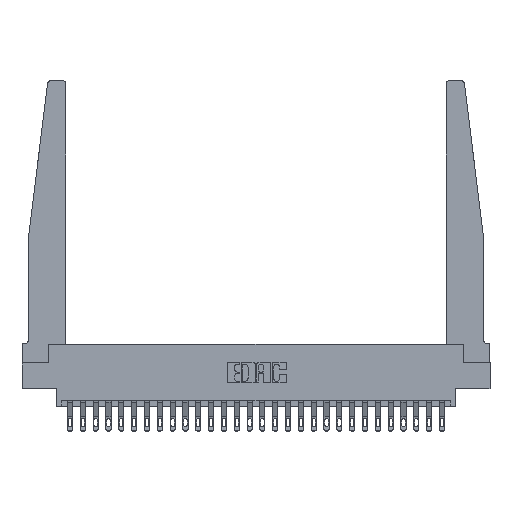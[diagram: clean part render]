
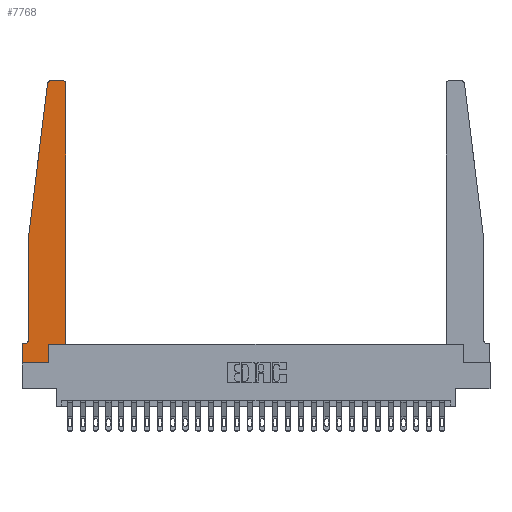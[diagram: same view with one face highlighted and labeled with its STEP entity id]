
A CAD part, top view. The second image highlights one B-rep face of the part: STEP entity #7768.
In plain terms, the highlighted planar face has unit normal (0, 0, 1).
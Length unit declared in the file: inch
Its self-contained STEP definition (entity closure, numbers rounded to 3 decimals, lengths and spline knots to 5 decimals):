
#263 = LINE ( 'NONE', #19004, #9302 ) ;
#421 = LINE ( 'NONE', #19478, #10753 ) ;
#685 = ORIENTED_EDGE ( 'NONE', *, *, #16748, .T. ) ;
#1182 = CARTESIAN_POINT ( 'NONE',  ( 0., 0., 0.37 ) ) ;
#1419 = EDGE_CURVE ( 'NONE', #20278, #16395, #15448, .T. ) ;
#1498 = ORIENTED_EDGE ( 'NONE', *, *, #15042, .T. ) ;
#1793 = EDGE_CURVE ( 'NONE', #17614, #8062, #23989, .T. ) ;
#1898 = VERTEX_POINT ( 'NONE', #14999 ) ;
#2315 = CARTESIAN_POINT ( 'NONE',  ( 0.065, 1.25, 0.37 ) ) ;
#2324 = VECTOR ( 'NONE', #16063, 39.37008 ) ;
#2696 = DIRECTION ( 'NONE',  ( 0., 0., 1. ) ) ;
#2909 = VECTOR ( 'NONE', #12685, 39.37008 ) ;
#3047 = CARTESIAN_POINT ( 'NONE',  ( 0.065, 1.25, 0.37 ) ) ;
#3545 = LINE ( 'NONE', #2315, #13821 ) ;
#3773 = ORIENTED_EDGE ( 'NONE', *, *, #16901, .T. ) ;
#3950 = CARTESIAN_POINT ( 'NONE',  ( 0.2605, 0.18, 0.37 ) ) ;
#3967 = CARTESIAN_POINT ( 'NONE',  ( 0.425, 0.18, 0.37 ) ) ;
#4061 = DIRECTION ( 'NONE',  ( 0., 0., 1. ) ) ;
#4295 = CARTESIAN_POINT ( 'NONE',  ( 0.425, 2.72, 0.37 ) ) ;
#4345 = CARTESIAN_POINT ( 'NONE',  ( 0.015, 0.1875, 0.37 ) ) ;
#4412 = DIRECTION ( 'NONE',  ( 0., -1., 0. ) ) ;
#4788 = CIRCLE ( 'NONE', #16052, 0.05 ) ;
#5064 = AXIS2_PLACEMENT_3D ( 'NONE', #16318, #4061, #18384 ) ;
#5149 = PLANE ( 'NONE',  #22748 ) ;
#6075 = CARTESIAN_POINT ( 'NONE',  ( 0.27653, 2.75, 0.37 ) ) ;
#6296 = CARTESIAN_POINT ( 'NONE',  ( 0.425, 0.18, 0.37 ) ) ;
#6361 = VERTEX_POINT ( 'NONE', #23131 ) ;
#7158 = EDGE_CURVE ( 'NONE', #16395, #17614, #421, .T. ) ;
#7190 = DIRECTION ( 'NONE',  ( 0., 0., 1. ) ) ;
#7486 = FACE_OUTER_BOUND ( 'NONE', #25118, .T. ) ;
#7745 = VERTEX_POINT ( 'NONE', #3047 ) ;
#7768 = ADVANCED_FACE ( 'NONE', ( #7486 ), #5149, .T. ) ;
#7907 = ORIENTED_EDGE ( 'NONE', *, *, #1419, .T. ) ;
#8062 = VERTEX_POINT ( 'NONE', #3950 ) ;
#8379 = DIRECTION ( 'NONE',  ( 0., 1., 0. ) ) ;
#8813 = DIRECTION ( 'NONE',  ( -1., 0., 0. ) ) ;
#9219 = DIRECTION ( 'NONE',  ( 0., 0., -1. ) ) ;
#9302 = VECTOR ( 'NONE', #8813, 39.37008 ) ;
#9306 = DIRECTION ( 'NONE',  ( 1., 0., 0. ) ) ;
#9968 = LINE ( 'NONE', #17650, #14748 ) ;
#10045 = CARTESIAN_POINT ( 'NONE',  ( 0.395, 2.75, 0.37 ) ) ;
#10150 = EDGE_CURVE ( 'NONE', #8062, #26365, #23854, .T. ) ;
#10352 = VECTOR ( 'NONE', #8379, 39.37008 ) ;
#10753 = VECTOR ( 'NONE', #9306, 39.37008 ) ;
#11346 = CIRCLE ( 'NONE', #5064, 0.03 ) ;
#11562 = CARTESIAN_POINT ( 'NONE',  ( 0.2605, 0., 0.37 ) ) ;
#12364 = EDGE_CURVE ( 'NONE', #25567, #20278, #13276, .T. ) ;
#12450 = EDGE_CURVE ( 'NONE', #18329, #1898, #11346, .T. ) ;
#12685 = DIRECTION ( 'NONE',  ( 0., 1., 0. ) ) ;
#13276 = LINE ( 'NONE', #14001, #2324 ) ;
#13690 = VECTOR ( 'NONE', #18285, 39.37008 ) ;
#13821 = VECTOR ( 'NONE', #4412, 39.37008 ) ;
#14001 = CARTESIAN_POINT ( 'NONE',  ( 0.065, 0.1875, 0.37 ) ) ;
#14748 = VECTOR ( 'NONE', #19721, 39.37008 ) ;
#14785 = CARTESIAN_POINT ( 'NONE',  ( 0.425, 0.18, 0.37 ) ) ;
#14952 = ORIENTED_EDGE ( 'NONE', *, *, #12364, .T. ) ;
#14992 = CARTESIAN_POINT ( 'NONE',  ( 0.395, 2.72, 0.37 ) ) ;
#14999 = CARTESIAN_POINT ( 'NONE',  ( 0.24675, 2.72367, 0.37 ) ) ;
#15042 = EDGE_CURVE ( 'NONE', #1898, #7745, #9968, .T. ) ;
#15448 = LINE ( 'NONE', #1182, #20854 ) ;
#15514 = EDGE_CURVE ( 'NONE', #20258, #18329, #263, .T. ) ;
#15560 = DIRECTION ( 'NONE',  ( 0., -1., 0. ) ) ;
#15766 = LINE ( 'NONE', #6296, #10352 ) ;
#16052 = AXIS2_PLACEMENT_3D ( 'NONE', #21433, #9219, #23465 ) ;
#16063 = DIRECTION ( 'NONE',  ( -1., 0., 0. ) ) ;
#16318 = CARTESIAN_POINT ( 'NONE',  ( 0.27653, 2.72, 0.37 ) ) ;
#16395 = VERTEX_POINT ( 'NONE', #21669 ) ;
#16451 = ORIENTED_EDGE ( 'NONE', *, *, #15514, .T. ) ;
#16748 = EDGE_CURVE ( 'NONE', #26365, #18403, #15766, .T. ) ;
#16901 = EDGE_CURVE ( 'NONE', #18403, #20258, #22099, .T. ) ;
#17042 = DIRECTION ( 'NONE',  ( 1., 0., 0. ) ) ;
#17256 = EDGE_CURVE ( 'NONE', #7745, #6361, #3545, .T. ) ;
#17403 = ORIENTED_EDGE ( 'NONE', *, *, #12450, .T. ) ;
#17614 = VERTEX_POINT ( 'NONE', #11562 ) ;
#17650 = CARTESIAN_POINT ( 'NONE',  ( 0.065, 1.25, 0.37 ) ) ;
#18244 = CARTESIAN_POINT ( 'NONE',  ( 0., 0.1875, 0.37 ) ) ;
#18285 = DIRECTION ( 'NONE',  ( 1., 0., 0. ) ) ;
#18329 = VERTEX_POINT ( 'NONE', #6075 ) ;
#18384 = DIRECTION ( 'NONE',  ( 1., 0., 0. ) ) ;
#18403 = VERTEX_POINT ( 'NONE', #4295 ) ;
#18653 = EDGE_CURVE ( 'NONE', #6361, #25567, #4788, .T. ) ;
#19004 = CARTESIAN_POINT ( 'NONE',  ( 0.25, 2.75, 0.37 ) ) ;
#19451 = CARTESIAN_POINT ( 'NONE',  ( 0., 0.1875, 0.37 ) ) ;
#19478 = CARTESIAN_POINT ( 'NONE',  ( 0., 0., 0.37 ) ) ;
#19721 = DIRECTION ( 'NONE',  ( -0.122, -0.992, 0. ) ) ;
#20139 = ORIENTED_EDGE ( 'NONE', *, *, #7158, .T. ) ;
#20258 = VERTEX_POINT ( 'NONE', #10045 ) ;
#20278 = VERTEX_POINT ( 'NONE', #18244 ) ;
#20854 = VECTOR ( 'NONE', #15560, 39.37008 ) ;
#21433 = CARTESIAN_POINT ( 'NONE',  ( 0.015, 0.2375, 0.37 ) ) ;
#21478 = DIRECTION ( 'NONE',  ( 1., 0., 0. ) ) ;
#21669 = CARTESIAN_POINT ( 'NONE',  ( 0., 0., 0.37 ) ) ;
#21936 = ORIENTED_EDGE ( 'NONE', *, *, #18653, .T. ) ;
#22099 = CIRCLE ( 'NONE', #23573, 0.03 ) ;
#22132 = ORIENTED_EDGE ( 'NONE', *, *, #17256, .T. ) ;
#22684 = ORIENTED_EDGE ( 'NONE', *, *, #1793, .T. ) ;
#22748 = AXIS2_PLACEMENT_3D ( 'NONE', #19451, #7190, #21478 ) ;
#23131 = CARTESIAN_POINT ( 'NONE',  ( 0.065, 0.2375, 0.37 ) ) ;
#23465 = DIRECTION ( 'NONE',  ( -1., 0., 0. ) ) ;
#23573 = AXIS2_PLACEMENT_3D ( 'NONE', #14992, #2696, #17042 ) ;
#23854 = LINE ( 'NONE', #3967, #13690 ) ;
#23989 = LINE ( 'NONE', #24833, #2909 ) ;
#24833 = CARTESIAN_POINT ( 'NONE',  ( 0.2605, 0.18, 0.37 ) ) ;
#25118 = EDGE_LOOP ( 'NONE', ( #16451, #17403, #1498, #22132, #21936, #14952, #7907, #20139, #22684, #25188, #685, #3773 ) ) ;
#25188 = ORIENTED_EDGE ( 'NONE', *, *, #10150, .T. ) ;
#25567 = VERTEX_POINT ( 'NONE', #4345 ) ;
#26365 = VERTEX_POINT ( 'NONE', #14785 ) ;
